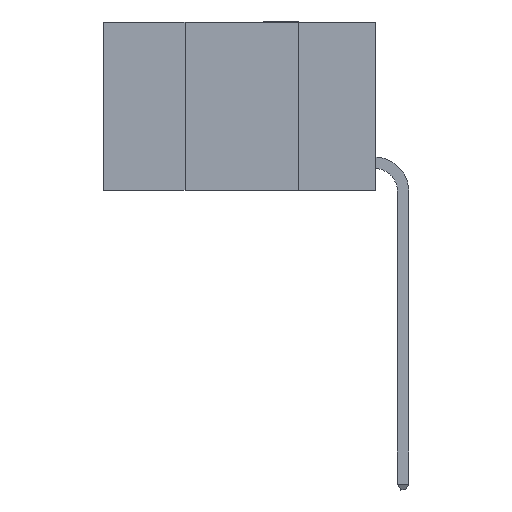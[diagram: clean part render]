
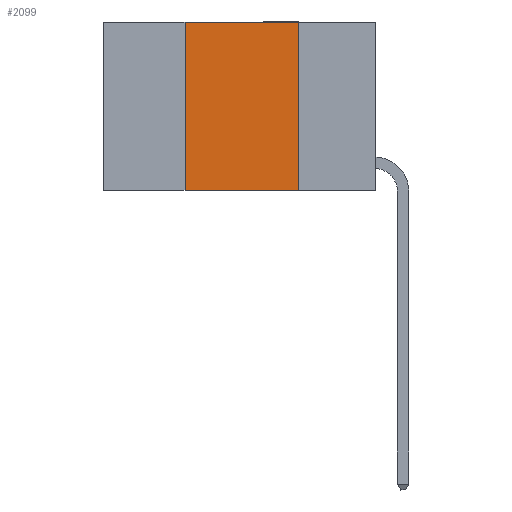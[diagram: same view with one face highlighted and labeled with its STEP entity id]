
A CAD part, left-side view. The second image highlights one B-rep face of the part: STEP entity #2099.
In plain terms, the highlighted planar face has unit normal (-1, 0, 0).
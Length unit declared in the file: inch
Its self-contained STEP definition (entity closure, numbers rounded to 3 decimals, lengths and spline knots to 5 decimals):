
#37 = ORIENTED_EDGE ( 'NONE', *, *, #5049, .F. ) ;
#174 = CARTESIAN_POINT ( 'NONE',  ( 0., 0.42, -0.37 ) ) ;
#183 = VERTEX_POINT ( 'NONE', #5060 ) ;
#449 = AXIS2_PLACEMENT_3D ( 'NONE', #8426, #1103, #3804 ) ;
#695 = EDGE_CURVE ( 'NONE', #4485, #183, #1994, .T. ) ;
#732 = CARTESIAN_POINT ( 'NONE',  ( 0., 0.17, 0. ) ) ;
#1090 = VECTOR ( 'NONE', #6359, 39.37008 ) ;
#1103 = DIRECTION ( 'NONE',  ( 1., 0., 0. ) ) ;
#1610 = VECTOR ( 'NONE', #7376, 39.37008 ) ;
#1994 = LINE ( 'NONE', #4709, #1610 ) ;
#2099 = ADVANCED_FACE ( 'NONE', ( #2480 ), #7112, .F. ) ;
#2160 = LINE ( 'NONE', #3655, #1090 ) ;
#2480 = FACE_OUTER_BOUND ( 'NONE', #6840, .T. ) ;
#2545 = LINE ( 'NONE', #732, #7494 ) ;
#2591 = VECTOR ( 'NONE', #5802, 39.37008 ) ;
#3655 = CARTESIAN_POINT ( 'NONE',  ( 0., 0.42, 0. ) ) ;
#3804 = DIRECTION ( 'NONE',  ( 0., 0., -1. ) ) ;
#4485 = VERTEX_POINT ( 'NONE', #174 ) ;
#4601 = VERTEX_POINT ( 'NONE', #4829 ) ;
#4709 = CARTESIAN_POINT ( 'NONE',  ( 0., 0.6, -0.37 ) ) ;
#4829 = CARTESIAN_POINT ( 'NONE',  ( 0., 0.42, 0. ) ) ;
#5049 = EDGE_CURVE ( 'NONE', #5113, #183, #2545, .T. ) ;
#5060 = CARTESIAN_POINT ( 'NONE',  ( 0., 0.17, -0.37 ) ) ;
#5113 = VERTEX_POINT ( 'NONE', #7767 ) ;
#5126 = ORIENTED_EDGE ( 'NONE', *, *, #8359, .F. ) ;
#5584 = EDGE_CURVE ( 'NONE', #4601, #5113, #6915, .T. ) ;
#5802 = DIRECTION ( 'NONE',  ( 0., -1., 0. ) ) ;
#6259 = CARTESIAN_POINT ( 'NONE',  ( 0., 0.6, 0. ) ) ;
#6344 = ORIENTED_EDGE ( 'NONE', *, *, #695, .T. ) ;
#6359 = DIRECTION ( 'NONE',  ( 0., 0., 1. ) ) ;
#6840 = EDGE_LOOP ( 'NONE', ( #37, #8570, #5126, #6344 ) ) ;
#6866 = DIRECTION ( 'NONE',  ( 0., 0., -1. ) ) ;
#6915 = LINE ( 'NONE', #6259, #2591 ) ;
#7112 = PLANE ( 'NONE',  #449 ) ;
#7376 = DIRECTION ( 'NONE',  ( 0., -1., 0. ) ) ;
#7494 = VECTOR ( 'NONE', #6866, 39.37008 ) ;
#7767 = CARTESIAN_POINT ( 'NONE',  ( 0., 0.17, 0. ) ) ;
#8359 = EDGE_CURVE ( 'NONE', #4485, #4601, #2160, .T. ) ;
#8426 = CARTESIAN_POINT ( 'NONE',  ( 0., 0.6, 0. ) ) ;
#8570 = ORIENTED_EDGE ( 'NONE', *, *, #5584, .F. ) ;
